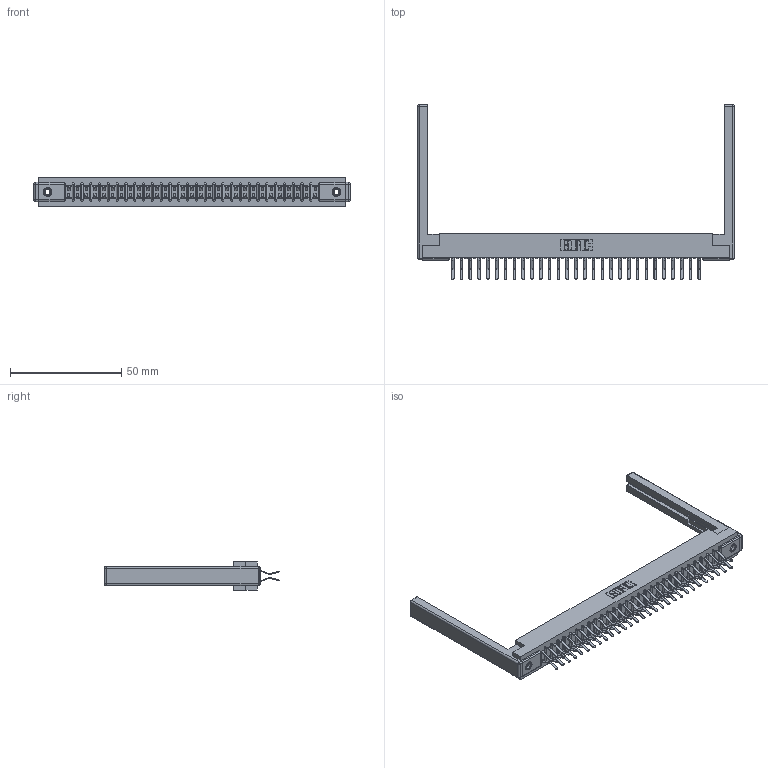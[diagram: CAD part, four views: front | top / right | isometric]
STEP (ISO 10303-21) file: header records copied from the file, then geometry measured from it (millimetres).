
FILE_DESCRIPTION (( 'STEP AP203' ), '1' );
FILE_NAME ('357-058-560-268.STEP', '2019-09-19T05:49:20', ( '' ), ( '' ), 'SwSTEP 2.0', 'SolidWorks 2016', '' );
FILE_SCHEMA (( 'CONFIG_CONTROL_DESIGN' ));
Length unit declared in the file: inch
Products named in the file (5): 357-058-560-268; 307-220-068; 307-290-001_560; 307 Part_.156 Dia Mounting Holes; 345-250-001_345-250-001-102
Assembly tree (63 placements, depth 2):
  357-058-560-268
    307 Part_.156 Dia Mounting Holes
    307-290-001_560  x58
    307-220-068  x2
    345-250-001_345-250-001-102  x2
Bounding box: 142.34 x 78.69 x 12.7 mm (x, y, z)
Volume: 19497.1 mm3; surface area: 22604.7 mm2
Topology: 63 solids, 63 shells, 3202 faces, 8949 edges, 5786 vertices
Faces by surface type: plane 2072, cylinder 1046, sphere 68, cone 12, torus 4
Entity records: 30255 total; most frequent: CARTESIAN_POINT 4930, ORIENTED_EDGE 4876, DIRECTION 4850, EDGE_CURVE 2438, VECTOR 1862, LINE 1862, VERTEX_POINT 1574, AXIS2_PLACEMENT_3D 1494
